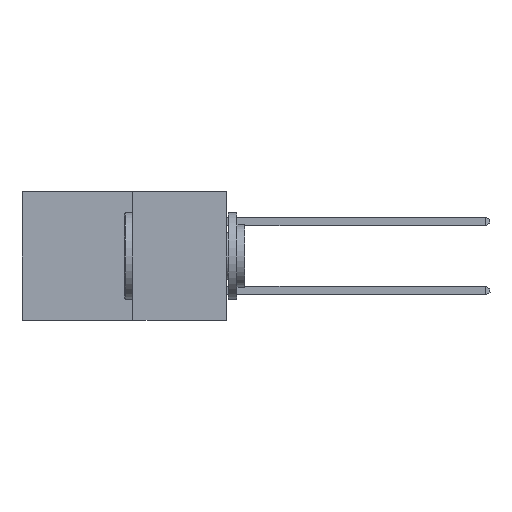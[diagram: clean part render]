
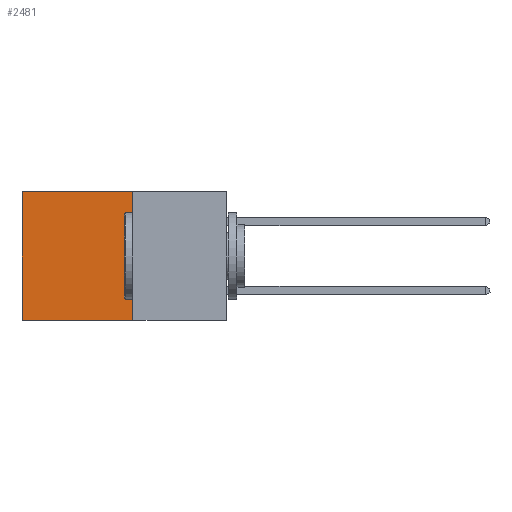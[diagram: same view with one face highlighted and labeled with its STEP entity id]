
A CAD part, left-side view. The second image highlights one B-rep face of the part: STEP entity #2481.
In plain terms, the highlighted planar face has unit normal (-1, 0, 0).
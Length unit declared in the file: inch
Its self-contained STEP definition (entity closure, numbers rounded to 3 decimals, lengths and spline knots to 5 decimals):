
#341 = CARTESIAN_POINT ( 'NONE',  ( 0.277, 0.59, 0. ) ) ;
#1723 = ORIENTED_EDGE ( 'NONE', *, *, #8241, .T. ) ;
#2045 = VECTOR ( 'NONE', #27950, 39.37008 ) ;
#2481 = ADVANCED_FACE ( 'NONE', ( #7318 ), #13990, .F. ) ;
#2891 = DIRECTION ( 'NONE',  ( 0., 1., 0. ) ) ;
#5691 = VECTOR ( 'NONE', #17593, 39.37008 ) ;
#5783 = ORIENTED_EDGE ( 'NONE', *, *, #16415, .F. ) ;
#5863 = DIRECTION ( 'NONE',  ( 0., 0., -1. ) ) ;
#6057 = CARTESIAN_POINT ( 'NONE',  ( 0.277, 0.59, -0.37 ) ) ;
#6428 = VECTOR ( 'NONE', #2891, 39.37008 ) ;
#6571 = ORIENTED_EDGE ( 'NONE', *, *, #21889, .F. ) ;
#6793 = VERTEX_POINT ( 'NONE', #341 ) ;
#7048 = VECTOR ( 'NONE', #5863, 39.37008 ) ;
#7318 = FACE_OUTER_BOUND ( 'NONE', #17727, .T. ) ;
#8059 = CARTESIAN_POINT ( 'NONE',  ( 0.277, 0.27, -0.37 ) ) ;
#8241 = EDGE_CURVE ( 'NONE', #15263, #6793, #27489, .T. ) ;
#8754 = CARTESIAN_POINT ( 'NONE',  ( 0.277, 0.27, -0.37 ) ) ;
#9066 = EDGE_CURVE ( 'NONE', #6793, #22868, #18668, .T. ) ;
#9537 = VERTEX_POINT ( 'NONE', #8059 ) ;
#13821 = LINE ( 'NONE', #14976, #2045 ) ;
#13990 = PLANE ( 'NONE',  #27385 ) ;
#14583 = ORIENTED_EDGE ( 'NONE', *, *, #9066, .T. ) ;
#14976 = CARTESIAN_POINT ( 'NONE',  ( 0.277, 0.27, -0.37 ) ) ;
#15263 = VERTEX_POINT ( 'NONE', #25076 ) ;
#16415 = EDGE_CURVE ( 'NONE', #15263, #9537, #13821, .T. ) ;
#17593 = DIRECTION ( 'NONE',  ( 0., 1., 0. ) ) ;
#17683 = CARTESIAN_POINT ( 'NONE',  ( 0.277, 0.27, 0. ) ) ;
#17727 = EDGE_LOOP ( 'NONE', ( #14583, #6571, #5783, #1723 ) ) ;
#18668 = LINE ( 'NONE', #6057, #7048 ) ;
#21889 = EDGE_CURVE ( 'NONE', #9537, #22868, #23169, .T. ) ;
#22167 = CARTESIAN_POINT ( 'NONE',  ( 0.277, 0.59, -0.37 ) ) ;
#22595 = DIRECTION ( 'NONE',  ( 1., 0., 0. ) ) ;
#22840 = DIRECTION ( 'NONE',  ( 0., 0., -1. ) ) ;
#22868 = VERTEX_POINT ( 'NONE', #22167 ) ;
#23169 = LINE ( 'NONE', #24857, #6428 ) ;
#24857 = CARTESIAN_POINT ( 'NONE',  ( 0.277, 0.27, -0.37 ) ) ;
#25076 = CARTESIAN_POINT ( 'NONE',  ( 0.277, 0.27, 0. ) ) ;
#27385 = AXIS2_PLACEMENT_3D ( 'NONE', #8754, #22595, #22840 ) ;
#27489 = LINE ( 'NONE', #17683, #5691 ) ;
#27950 = DIRECTION ( 'NONE',  ( 0., 0., -1. ) ) ;
